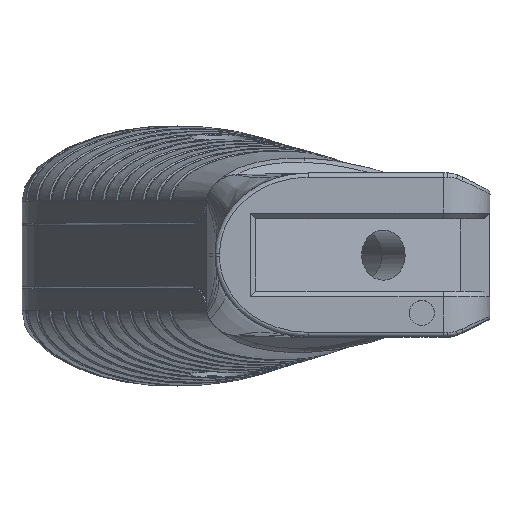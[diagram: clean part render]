
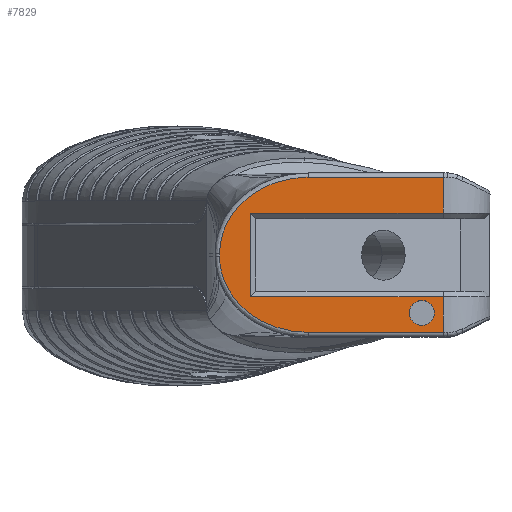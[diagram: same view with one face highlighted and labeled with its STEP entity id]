
A CAD part, top view. The second image highlights one B-rep face of the part: STEP entity #7829.
In plain terms, the highlighted planar face has unit normal (0, 0, 1).
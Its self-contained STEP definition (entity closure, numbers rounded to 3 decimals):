
#330=FACE_BOUND('',#2197,.T.);
#478=CIRCLE('',#8348,1.7);
#1084=B_SPLINE_CURVE_WITH_KNOTS('',3,(#51384,#51385,#51386,#51387,#51388,
#51389,#51390,#51391,#51392,#51393),.UNSPECIFIED.,.F.,.F.,(4,2,2,2,4),(0.,
0.571,0.976,1.452,1.75),
 .UNSPECIFIED.);
#1085=B_SPLINE_CURVE_WITH_KNOTS('',3,(#51396,#51397,#51398,#51399,#51400,
#51401,#51402,#51403,#51404,#51405,#51406,#51407,#51408,#51409),
 .UNSPECIFIED.,.F.,.F.,(4,2,2,2,2,2,4),(0.,0.148,0.479,
0.833,1.137,1.486,1.752),
 .UNSPECIFIED.);
#1283=PLANE('',#8347);
#1685=FACE_OUTER_BOUND('',#2196,.T.);
#2196=EDGE_LOOP('',(#6855,#6856,#6857,#6858,#6859,#6860,#6861,#6862,#6863,
#6864));
#2197=EDGE_LOOP('',(#6865));
#2606=LINE('',#51245,#2918);
#2611=LINE('',#51373,#2923);
#2612=LINE('',#51375,#2924);
#2613=LINE('',#51377,#2925);
#2614=LINE('',#51379,#2926);
#2615=LINE('',#51380,#2927);
#2616=LINE('',#51382,#2928);
#2617=LINE('',#51395,#2929);
#2918=VECTOR('',#9488,10.);
#2923=VECTOR('',#9509,10.);
#2924=VECTOR('',#9510,10.);
#2925=VECTOR('',#9511,10.);
#2926=VECTOR('',#9512,10.);
#2927=VECTOR('',#9513,10.);
#2928=VECTOR('',#9514,10.);
#2929=VECTOR('',#9515,10.);
#3593=VERTEX_POINT('',#51241);
#3595=VERTEX_POINT('',#51244);
#3611=VERTEX_POINT('',#51371);
#3612=VERTEX_POINT('',#51372);
#3613=VERTEX_POINT('',#51374);
#3614=VERTEX_POINT('',#51376);
#3615=VERTEX_POINT('',#51378);
#3616=VERTEX_POINT('',#51381);
#3617=VERTEX_POINT('',#51383);
#3618=VERTEX_POINT('',#51394);
#3619=VERTEX_POINT('',#51410);
#4698=EDGE_CURVE('',#3593,#3595,#2606,.T.);
#4716=EDGE_CURVE('',#3611,#3612,#2611,.T.);
#4717=EDGE_CURVE('',#3611,#3613,#2612,.T.);
#4718=EDGE_CURVE('',#3614,#3613,#2613,.T.);
#4719=EDGE_CURVE('',#3615,#3614,#2614,.T.);
#4720=EDGE_CURVE('',#3595,#3615,#2615,.T.);
#4721=EDGE_CURVE('',#3616,#3593,#2616,.T.);
#4722=EDGE_CURVE('',#3617,#3616,#1084,.T.);
#4723=EDGE_CURVE('',#3618,#3617,#2617,.T.);
#4724=EDGE_CURVE('',#3612,#3618,#1085,.T.);
#4725=EDGE_CURVE('',#3619,#3619,#478,.T.);
#6855=ORIENTED_EDGE('',*,*,#4716,.F.);
#6856=ORIENTED_EDGE('',*,*,#4717,.T.);
#6857=ORIENTED_EDGE('',*,*,#4718,.F.);
#6858=ORIENTED_EDGE('',*,*,#4719,.F.);
#6859=ORIENTED_EDGE('',*,*,#4720,.F.);
#6860=ORIENTED_EDGE('',*,*,#4698,.F.);
#6861=ORIENTED_EDGE('',*,*,#4721,.F.);
#6862=ORIENTED_EDGE('',*,*,#4722,.F.);
#6863=ORIENTED_EDGE('',*,*,#4723,.F.);
#6864=ORIENTED_EDGE('',*,*,#4724,.F.);
#6865=ORIENTED_EDGE('',*,*,#4725,.T.);
#7829=ADVANCED_FACE('',(#1685,#330),#1283,.T.);
#8347=AXIS2_PLACEMENT_3D('',#51370,#9507,#9508);
#8348=AXIS2_PLACEMENT_3D('',#51411,#9516,#9517);
#9488=DIRECTION('',(0.,-1.,0.));
#9507=DIRECTION('center_axis',(0.,0.,
1.));
#9508=DIRECTION('ref_axis',(1.,0.,0.));
#9509=DIRECTION('',(-1.,0.,0.));
#9510=DIRECTION('',(0.,1.,0.));
#9511=DIRECTION('',(1.,0.,0.));
#9512=DIRECTION('',(0.,-1.,0.));
#9513=DIRECTION('',(-1.,0.,0.));
#9514=DIRECTION('',(1.,0.,0.));
#9515=DIRECTION('',(0.,1.,0.));
#9516=DIRECTION('center_axis',(0.,0.,
-1.));
#9517=DIRECTION('ref_axis',(0.,1.,0.));
#51241=CARTESIAN_POINT('',(-3.41,-21.904,42.306));
#51244=CARTESIAN_POINT('',(-3.41,-26.753,42.306));
#51245=CARTESIAN_POINT('',(-3.41,-37.292,42.306));
#51370=CARTESIAN_POINT('Origin',(-34.254,-37.291,42.305));
#51371=CARTESIAN_POINT('',(-3.41,-42.931,42.306));
#51372=CARTESIAN_POINT('',(-21.731,-42.931,42.306));
#51373=CARTESIAN_POINT('',(-27.992,-42.93,42.305));
#51374=CARTESIAN_POINT('',(-3.41,-38.082,42.306));
#51375=CARTESIAN_POINT('',(-3.41,-27.543,42.306));
#51376=CARTESIAN_POINT('',(-29.56,-38.081,42.305));
#51377=CARTESIAN_POINT('',(-32.259,-38.081,42.305));
#51378=CARTESIAN_POINT('',(-29.56,-26.753,42.305));
#51379=CARTESIAN_POINT('',(-29.56,-32.326,42.305));
#51380=CARTESIAN_POINT('',(-32.259,-26.753,42.305));
#51381=CARTESIAN_POINT('',(-21.73,-21.904,42.306));
#51382=CARTESIAN_POINT('',(-21.522,-21.904,42.306));
#51383=CARTESIAN_POINT('',(-33.751,-32.254,42.305));
#51384=CARTESIAN_POINT('Ctrl Pts',(-33.751,-32.254,
42.305));
#51385=CARTESIAN_POINT('Ctrl Pts',(-33.751,-30.35,
42.305));
#51386=CARTESIAN_POINT('Ctrl Pts',(-33.115,-28.459,
42.305));
#51387=CARTESIAN_POINT('Ctrl Pts',(-31.224,-25.776,
42.305));
#51388=CARTESIAN_POINT('Ctrl Pts',(-30.229,-24.833,42.305));
#51389=CARTESIAN_POINT('Ctrl Pts',(-27.763,-23.186,
42.305));
#51390=CARTESIAN_POINT('Ctrl Pts',(-26.27,-22.57,
42.305));
#51391=CARTESIAN_POINT('Ctrl Pts',(-23.726,-22.011,
42.306));
#51392=CARTESIAN_POINT('Ctrl Pts',(-22.722,-21.904,
42.306));
#51393=CARTESIAN_POINT('Ctrl Pts',(-21.73,-21.904,
42.306));
#51394=CARTESIAN_POINT('',(-33.751,-32.58,42.305));
#51395=CARTESIAN_POINT('',(-33.751,-34.773,42.305));
#51396=CARTESIAN_POINT('Ctrl Pts',(-21.731,-42.931,
42.306));
#51397=CARTESIAN_POINT('Ctrl Pts',(-22.224,-42.93,
42.306));
#51398=CARTESIAN_POINT('Ctrl Pts',(-22.719,-42.904,
42.306));
#51399=CARTESIAN_POINT('Ctrl Pts',(-24.31,-42.734,42.306));
#51400=CARTESIAN_POINT('Ctrl Pts',(-25.392,-42.486,
42.305));
#51401=CARTESIAN_POINT('Ctrl Pts',(-27.545,-41.698,
42.305));
#51402=CARTESIAN_POINT('Ctrl Pts',(-28.603,-41.14,
42.305));
#51403=CARTESIAN_POINT('Ctrl Pts',(-30.381,-39.825,
42.305));
#51404=CARTESIAN_POINT('Ctrl Pts',(-31.115,-39.117,
42.305));
#51405=CARTESIAN_POINT('Ctrl Pts',(-32.454,-37.386,
42.305));
#51406=CARTESIAN_POINT('Ctrl Pts',(-33.011,-36.336,
42.305));
#51407=CARTESIAN_POINT('Ctrl Pts',(-33.615,-34.364,
42.305));
#51408=CARTESIAN_POINT('Ctrl Pts',(-33.751,-33.466,
42.305));
#51409=CARTESIAN_POINT('Ctrl Pts',(-33.751,-32.58,
42.305));
#51410=CARTESIAN_POINT('',(-6.305,-41.994,42.306));
#51411=CARTESIAN_POINT('Origin',(-6.305,-40.294,42.306));
